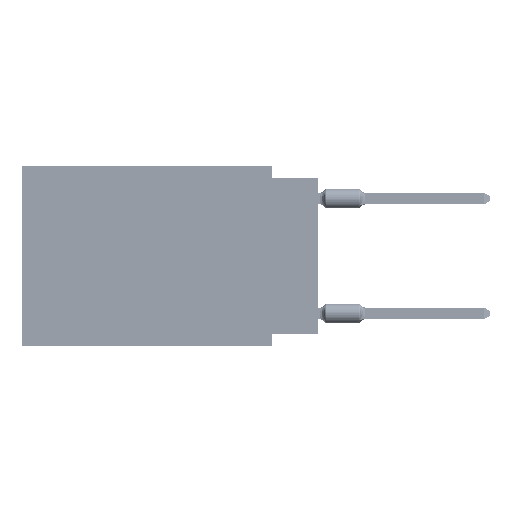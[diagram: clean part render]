
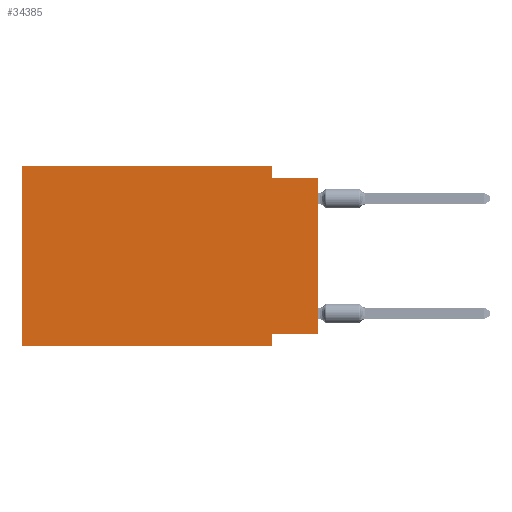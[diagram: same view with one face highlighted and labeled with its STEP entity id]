
A CAD part, left-side view. The second image highlights one B-rep face of the part: STEP entity #34385.
In plain terms, the highlighted planar face has unit normal (-1, 0, 0).
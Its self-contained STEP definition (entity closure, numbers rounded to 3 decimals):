
#634 = VERTEX_POINT ( 'NONE', #14428 ) ;
#3173 = VERTEX_POINT ( 'NONE', #43504 ) ;
#6233 = CARTESIAN_POINT ( 'NONE',  ( 0., 16.383, 0. ) ) ;
#6804 = CARTESIAN_POINT ( 'NONE',  ( 0., 16.383, -9.906 ) ) ;
#7950 = VECTOR ( 'NONE', #16710, 1000. ) ;
#8212 = VERTEX_POINT ( 'NONE', #35887 ) ;
#9736 = DIRECTION ( 'NONE',  ( 1., 0., 0. ) ) ;
#10279 = AXIS2_PLACEMENT_3D ( 'NONE', #59169, #9736, #25732 ) ;
#10356 = ORIENTED_EDGE ( 'NONE', *, *, #34063, .T. ) ;
#10624 = LINE ( 'NONE', #37876, #49306 ) ;
#12587 = EDGE_CURVE ( 'NONE', #28004, #634, #18060, .T. ) ;
#14428 = CARTESIAN_POINT ( 'NONE',  ( 0., 2.54, -9.906 ) ) ;
#14452 = DIRECTION ( 'NONE',  ( 0., -1., 0. ) ) ;
#16710 = DIRECTION ( 'NONE',  ( 0., 0., 1. ) ) ;
#16999 = VECTOR ( 'NONE', #34569, 1000. ) ;
#18060 = LINE ( 'NONE', #6804, #44543 ) ;
#18975 = CARTESIAN_POINT ( 'NONE',  ( 0., 2.54, -9.271 ) ) ;
#19243 = EDGE_CURVE ( 'NONE', #3173, #36562, #20992, .T. ) ;
#19880 = ORIENTED_EDGE ( 'NONE', *, *, #30355, .F. ) ;
#20654 = FACE_OUTER_BOUND ( 'NONE', #60707, .T. ) ;
#20977 = CARTESIAN_POINT ( 'NONE',  ( 0., 0., -0.635 ) ) ;
#20992 = LINE ( 'NONE', #41729, #24141 ) ;
#21250 = LINE ( 'NONE', #61547, #37243 ) ;
#21480 = VECTOR ( 'NONE', #59602, 1000. ) ;
#22819 = VECTOR ( 'NONE', #50099, 1000. ) ;
#23913 = ORIENTED_EDGE ( 'NONE', *, *, #25065, .F. ) ;
#24141 = VECTOR ( 'NONE', #14452, 1000. ) ;
#25065 = EDGE_CURVE ( 'NONE', #36562, #8212, #21250, .T. ) ;
#25732 = DIRECTION ( 'NONE',  ( 0., 0., -1. ) ) ;
#26713 = DIRECTION ( 'NONE',  ( 0., 0., -1. ) ) ;
#28004 = VERTEX_POINT ( 'NONE', #34155 ) ;
#28625 = CARTESIAN_POINT ( 'NONE',  ( 0., 0., -9.271 ) ) ;
#28889 = VERTEX_POINT ( 'NONE', #54435 ) ;
#29812 = EDGE_CURVE ( 'NONE', #71567, #634, #10624, .T. ) ;
#30355 = EDGE_CURVE ( 'NONE', #8212, #57694, #42911, .T. ) ;
#31978 = CARTESIAN_POINT ( 'NONE',  ( 0., 0., -0.635 ) ) ;
#33501 = DIRECTION ( 'NONE',  ( 0., 0., -1. ) ) ;
#34063 = EDGE_CURVE ( 'NONE', #28889, #57694, #38160, .T. ) ;
#34155 = CARTESIAN_POINT ( 'NONE',  ( 0., 16.383, -9.906 ) ) ;
#34385 = ADVANCED_FACE ( 'NONE', ( #20654 ), #41748, .F. ) ;
#34569 = DIRECTION ( 'NONE',  ( 0., 0., 1. ) ) ;
#35887 = CARTESIAN_POINT ( 'NONE',  ( 0., 2.54, -0.635 ) ) ;
#36562 = VERTEX_POINT ( 'NONE', #37556 ) ;
#37243 = VECTOR ( 'NONE', #26713, 1000. ) ;
#37556 = CARTESIAN_POINT ( 'NONE',  ( 0., 2.54, 0. ) ) ;
#37876 = CARTESIAN_POINT ( 'NONE',  ( 0., 2.54, -9.906 ) ) ;
#38160 = LINE ( 'NONE', #55590, #7950 ) ;
#38457 = LINE ( 'NONE', #28625, #22819 ) ;
#38962 = EDGE_CURVE ( 'NONE', #28889, #71567, #38457, .T. ) ;
#40020 = LINE ( 'NONE', #6233, #16999 ) ;
#40604 = DIRECTION ( 'NONE',  ( 0., -1., 0. ) ) ;
#41729 = CARTESIAN_POINT ( 'NONE',  ( 0., 16.383, 0. ) ) ;
#41748 = PLANE ( 'NONE',  #10279 ) ;
#42911 = LINE ( 'NONE', #31978, #21480 ) ;
#43504 = CARTESIAN_POINT ( 'NONE',  ( 0., 16.383, 0. ) ) ;
#44308 = ORIENTED_EDGE ( 'NONE', *, *, #38962, .F. ) ;
#44543 = VECTOR ( 'NONE', #40604, 1000. ) ;
#48970 = ORIENTED_EDGE ( 'NONE', *, *, #19243, .F. ) ;
#49306 = VECTOR ( 'NONE', #33501, 1000. ) ;
#50099 = DIRECTION ( 'NONE',  ( 0., 1., 0. ) ) ;
#53393 = ORIENTED_EDGE ( 'NONE', *, *, #12587, .T. ) ;
#53422 = EDGE_CURVE ( 'NONE', #28004, #3173, #40020, .T. ) ;
#54435 = CARTESIAN_POINT ( 'NONE',  ( 0., 0., -9.271 ) ) ;
#55590 = CARTESIAN_POINT ( 'NONE',  ( 0., 0., 0. ) ) ;
#57694 = VERTEX_POINT ( 'NONE', #20977 ) ;
#58502 = ORIENTED_EDGE ( 'NONE', *, *, #53422, .F. ) ;
#59169 = CARTESIAN_POINT ( 'NONE',  ( 0., 16.383, 0. ) ) ;
#59602 = DIRECTION ( 'NONE',  ( 0., -1., 0. ) ) ;
#60707 = EDGE_LOOP ( 'NONE', ( #10356, #19880, #23913, #48970, #58502, #53393, #67814, #44308 ) ) ;
#61547 = CARTESIAN_POINT ( 'NONE',  ( 0., 2.54, 0. ) ) ;
#67814 = ORIENTED_EDGE ( 'NONE', *, *, #29812, .F. ) ;
#71567 = VERTEX_POINT ( 'NONE', #18975 ) ;
